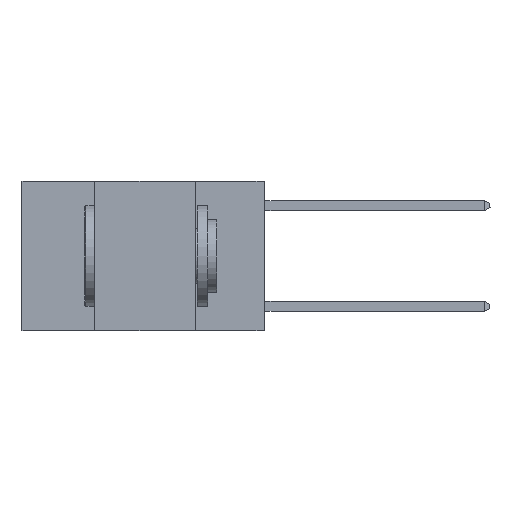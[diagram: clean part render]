
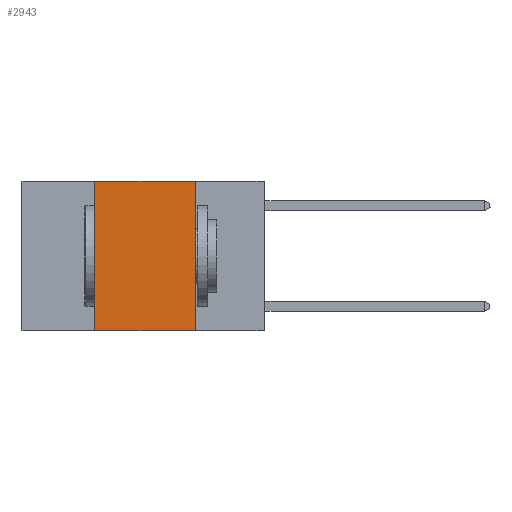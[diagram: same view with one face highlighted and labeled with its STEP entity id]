
A CAD part, left-side view. The second image highlights one B-rep face of the part: STEP entity #2943.
In plain terms, the highlighted planar face has unit normal (-1, 0, 0).
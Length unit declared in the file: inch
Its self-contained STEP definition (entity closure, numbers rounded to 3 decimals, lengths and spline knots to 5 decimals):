
#2779 = DIRECTION ( 'NONE',  ( 1., 0., 0. ) ) ;
#2943 = ADVANCED_FACE ( 'NONE', ( #19486 ), #24409, .F. ) ;
#3324 = EDGE_CURVE ( 'NONE', #22182, #20460, #16675, .T. ) ;
#3556 = CARTESIAN_POINT ( 'NONE',  ( 0., 0.42, -0.37 ) ) ;
#5232 = LINE ( 'NONE', #7905, #21030 ) ;
#6779 = CARTESIAN_POINT ( 'NONE',  ( 0., 0.6, 0. ) ) ;
#7275 = VERTEX_POINT ( 'NONE', #19456 ) ;
#7905 = CARTESIAN_POINT ( 'NONE',  ( 0., 0.6, -0.37 ) ) ;
#7922 = DIRECTION ( 'NONE',  ( 0., 0., -1. ) ) ;
#8485 = ORIENTED_EDGE ( 'NONE', *, *, #22871, .F. ) ;
#8680 = EDGE_CURVE ( 'NONE', #15918, #7275, #11216, .T. ) ;
#8783 = DIRECTION ( 'NONE',  ( 0., -1., 0. ) ) ;
#9607 = AXIS2_PLACEMENT_3D ( 'NONE', #12699, #2779, #16644 ) ;
#10092 = CARTESIAN_POINT ( 'NONE',  ( 0., 0.42, 0. ) ) ;
#10831 = VECTOR ( 'NONE', #7922, 39.37008 ) ;
#11117 = EDGE_LOOP ( 'NONE', ( #14730, #8485, #18972, #23051 ) ) ;
#11216 = LINE ( 'NONE', #10092, #20453 ) ;
#11838 = EDGE_CURVE ( 'NONE', #15918, #20460, #5232, .T. ) ;
#12699 = CARTESIAN_POINT ( 'NONE',  ( 0., 0.6, 0. ) ) ;
#13466 = CARTESIAN_POINT ( 'NONE',  ( 0., 0.17, -0.37 ) ) ;
#14730 = ORIENTED_EDGE ( 'NONE', *, *, #3324, .F. ) ;
#15918 = VERTEX_POINT ( 'NONE', #3556 ) ;
#16644 = DIRECTION ( 'NONE',  ( 0., 0., -1. ) ) ;
#16650 = CARTESIAN_POINT ( 'NONE',  ( 0., 0.17, 0. ) ) ;
#16675 = LINE ( 'NONE', #17768, #10831 ) ;
#17768 = CARTESIAN_POINT ( 'NONE',  ( 0., 0.17, 0. ) ) ;
#18972 = ORIENTED_EDGE ( 'NONE', *, *, #8680, .F. ) ;
#19448 = LINE ( 'NONE', #6779, #23473 ) ;
#19456 = CARTESIAN_POINT ( 'NONE',  ( 0., 0.42, 0. ) ) ;
#19486 = FACE_OUTER_BOUND ( 'NONE', #11117, .T. ) ;
#19737 = DIRECTION ( 'NONE',  ( 0., -1., 0. ) ) ;
#20453 = VECTOR ( 'NONE', #23970, 39.37008 ) ;
#20460 = VERTEX_POINT ( 'NONE', #13466 ) ;
#21030 = VECTOR ( 'NONE', #19737, 39.37008 ) ;
#22182 = VERTEX_POINT ( 'NONE', #16650 ) ;
#22871 = EDGE_CURVE ( 'NONE', #7275, #22182, #19448, .T. ) ;
#23051 = ORIENTED_EDGE ( 'NONE', *, *, #11838, .T. ) ;
#23473 = VECTOR ( 'NONE', #8783, 39.37008 ) ;
#23970 = DIRECTION ( 'NONE',  ( 0., 0., 1. ) ) ;
#24409 = PLANE ( 'NONE',  #9607 ) ;
